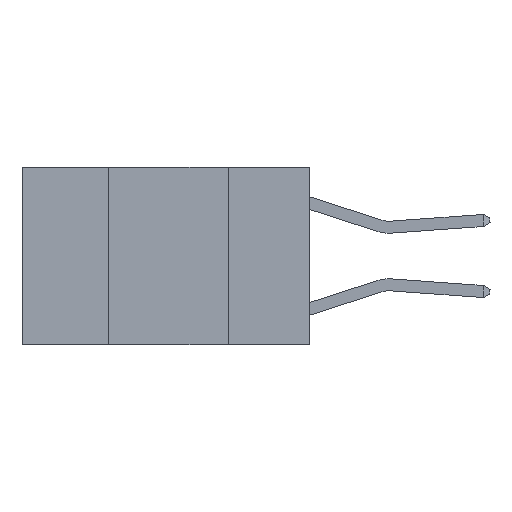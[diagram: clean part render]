
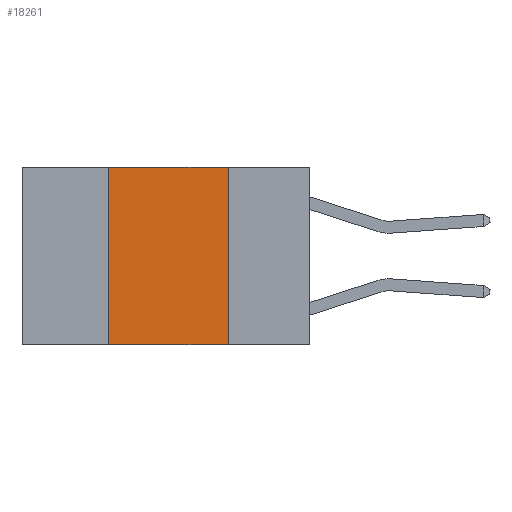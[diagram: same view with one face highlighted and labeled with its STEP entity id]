
A CAD part, left-side view. The second image highlights one B-rep face of the part: STEP entity #18261.
In plain terms, the highlighted planar face has unit normal (-1, 0, 0).
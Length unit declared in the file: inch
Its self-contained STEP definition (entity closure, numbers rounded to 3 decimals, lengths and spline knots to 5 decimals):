
#45 = EDGE_CURVE ( 'NONE', #3889, #7564, #16139, .T. ) ;
#139 = PLANE ( 'NONE',  #16898 ) ;
#1682 = CARTESIAN_POINT ( 'NONE',  ( 0., 0.42, 0. ) ) ;
#2541 = EDGE_CURVE ( 'NONE', #3889, #4830, #10486, .T. ) ;
#3746 = LINE ( 'NONE', #4203, #18326 ) ;
#3889 = VERTEX_POINT ( 'NONE', #13064 ) ;
#4203 = CARTESIAN_POINT ( 'NONE',  ( 0., 0.17, 0. ) ) ;
#4830 = VERTEX_POINT ( 'NONE', #1682 ) ;
#5450 = DIRECTION ( 'NONE',  ( 0., 0., -1. ) ) ;
#5811 = DIRECTION ( 'NONE',  ( 0., 0., -1. ) ) ;
#5912 = EDGE_LOOP ( 'NONE', ( #17908, #11257, #9031, #22648 ) ) ;
#6294 = CARTESIAN_POINT ( 'NONE',  ( 0., 0.17, 0. ) ) ;
#6719 = CARTESIAN_POINT ( 'NONE',  ( 0., 0.17, -0.37 ) ) ;
#7564 = VERTEX_POINT ( 'NONE', #6719 ) ;
#8372 = VERTEX_POINT ( 'NONE', #6294 ) ;
#8622 = DIRECTION ( 'NONE',  ( 0., -1., 0. ) ) ;
#8785 = DIRECTION ( 'NONE',  ( 0., 0., 1. ) ) ;
#9031 = ORIENTED_EDGE ( 'NONE', *, *, #2541, .F. ) ;
#9190 = FACE_OUTER_BOUND ( 'NONE', #5912, .T. ) ;
#10486 = LINE ( 'NONE', #17757, #12929 ) ;
#10525 = VECTOR ( 'NONE', #12931, 39.37008 ) ;
#10967 = VECTOR ( 'NONE', #8622, 39.37008 ) ;
#11257 = ORIENTED_EDGE ( 'NONE', *, *, #16810, .F. ) ;
#12682 = CARTESIAN_POINT ( 'NONE',  ( 0., 0.6, -0.37 ) ) ;
#12929 = VECTOR ( 'NONE', #8785, 39.37008 ) ;
#12931 = DIRECTION ( 'NONE',  ( 0., -1., 0. ) ) ;
#13064 = CARTESIAN_POINT ( 'NONE',  ( 0., 0.42, -0.37 ) ) ;
#14254 = CARTESIAN_POINT ( 'NONE',  ( 0., 0.6, 0. ) ) ;
#16139 = LINE ( 'NONE', #12682, #10525 ) ;
#16810 = EDGE_CURVE ( 'NONE', #4830, #8372, #19118, .T. ) ;
#16898 = AXIS2_PLACEMENT_3D ( 'NONE', #14254, #21323, #5450 ) ;
#17383 = CARTESIAN_POINT ( 'NONE',  ( 0., 0.6, 0. ) ) ;
#17757 = CARTESIAN_POINT ( 'NONE',  ( 0., 0.42, 0. ) ) ;
#17908 = ORIENTED_EDGE ( 'NONE', *, *, #22108, .F. ) ;
#18261 = ADVANCED_FACE ( 'NONE', ( #9190 ), #139, .F. ) ;
#18326 = VECTOR ( 'NONE', #5811, 39.37008 ) ;
#19118 = LINE ( 'NONE', #17383, #10967 ) ;
#21323 = DIRECTION ( 'NONE',  ( 1., 0., 0. ) ) ;
#22108 = EDGE_CURVE ( 'NONE', #8372, #7564, #3746, .T. ) ;
#22648 = ORIENTED_EDGE ( 'NONE', *, *, #45, .T. ) ;
